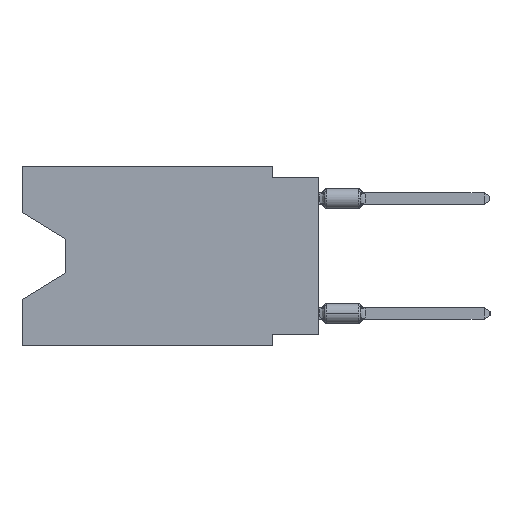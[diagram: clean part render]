
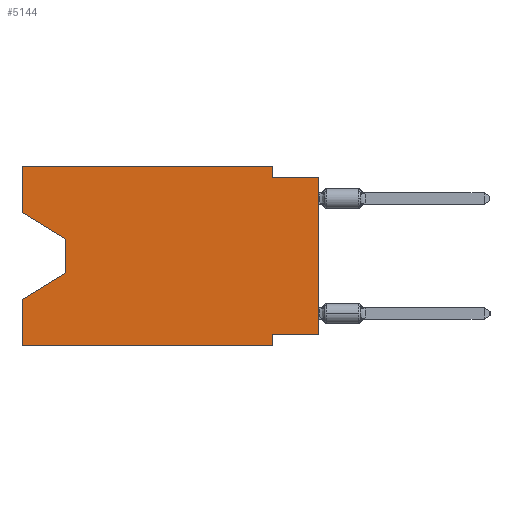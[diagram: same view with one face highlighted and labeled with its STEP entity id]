
A CAD part, left-side view. The second image highlights one B-rep face of the part: STEP entity #5144.
In plain terms, the highlighted planar face has unit normal (-1, 0, 0).
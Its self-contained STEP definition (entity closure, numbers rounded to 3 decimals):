
#274 = LINE ( 'NONE', #11532, #1977 ) ;
#690 = DIRECTION ( 'NONE',  ( 0., 0., -1. ) ) ;
#1440 = CARTESIAN_POINT ( 'NONE',  ( 0., 16.383, 0. ) ) ;
#1747 = VECTOR ( 'NONE', #36824, 1000. ) ;
#1977 = VECTOR ( 'NONE', #26783, 1000. ) ;
#3202 = EDGE_CURVE ( 'NONE', #27987, #41199, #40570, .T. ) ;
#3304 = LINE ( 'NONE', #14578, #1747 ) ;
#3527 = EDGE_CURVE ( 'NONE', #44847, #47909, #17283, .T. ) ;
#3804 = CARTESIAN_POINT ( 'NONE',  ( 0., 16.383, -7.36 ) ) ;
#4261 = VERTEX_POINT ( 'NONE', #49409 ) ;
#4263 = DIRECTION ( 'NONE',  ( 1., 0., 0. ) ) ;
#5144 = ADVANCED_FACE ( 'NONE', ( #42731 ), #8276, .F. ) ;
#5632 = EDGE_CURVE ( 'NONE', #35108, #4261, #16679, .T. ) ;
#5953 = CARTESIAN_POINT ( 'NONE',  ( 0., 16.383, -2.546 ) ) ;
#6007 = ORIENTED_EDGE ( 'NONE', *, *, #3527, .T. ) ;
#6340 = DIRECTION ( 'NONE',  ( 0., 0.855, -0.519 ) ) ;
#6975 = VERTEX_POINT ( 'NONE', #19221 ) ;
#7134 = ORIENTED_EDGE ( 'NONE', *, *, #3202, .T. ) ;
#7658 = EDGE_CURVE ( 'NONE', #43015, #47909, #18131, .T. ) ;
#8276 = PLANE ( 'NONE',  #19387 ) ;
#8695 = ORIENTED_EDGE ( 'NONE', *, *, #27275, .F. ) ;
#9591 = DIRECTION ( 'NONE',  ( 0., 0., 1. ) ) ;
#10071 = DIRECTION ( 'NONE',  ( 0., -1., 0. ) ) ;
#10151 = CARTESIAN_POINT ( 'NONE',  ( 0., 0., -0.635 ) ) ;
#10322 = CARTESIAN_POINT ( 'NONE',  ( 0., 2.54, 0. ) ) ;
#10509 = VECTOR ( 'NONE', #36534, 1000. ) ;
#11367 = CARTESIAN_POINT ( 'NONE',  ( 0., 2.54, -0.635 ) ) ;
#11532 = CARTESIAN_POINT ( 'NONE',  ( 0., 0., -9.271 ) ) ;
#12652 = VECTOR ( 'NONE', #44553, 1000. ) ;
#13189 = DIRECTION ( 'NONE',  ( 0., -1., 0. ) ) ;
#13385 = VECTOR ( 'NONE', #35360, 1000. ) ;
#13936 = CARTESIAN_POINT ( 'NONE',  ( 0., 16.383, -9.906 ) ) ;
#14056 = VERTEX_POINT ( 'NONE', #26756 ) ;
#14578 = CARTESIAN_POINT ( 'NONE',  ( 0., 16.383, 0. ) ) ;
#15410 = VECTOR ( 'NONE', #47177, 1000. ) ;
#15862 = ORIENTED_EDGE ( 'NONE', *, *, #24168, .T. ) ;
#16679 = LINE ( 'NONE', #47900, #18632 ) ;
#17283 = LINE ( 'NONE', #47758, #10509 ) ;
#17324 = CARTESIAN_POINT ( 'NONE',  ( 0., 2.54, 0. ) ) ;
#17822 = LINE ( 'NONE', #44307, #26389 ) ;
#17897 = DIRECTION ( 'NONE',  ( 0., -1., 0. ) ) ;
#18131 = LINE ( 'NONE', #10151, #45572 ) ;
#18632 = VECTOR ( 'NONE', #13189, 1000. ) ;
#19221 = CARTESIAN_POINT ( 'NONE',  ( 0., 16.383, -2.546 ) ) ;
#19224 = EDGE_CURVE ( 'NONE', #35108, #41199, #3304, .T. ) ;
#19387 = AXIS2_PLACEMENT_3D ( 'NONE', #23268, #4263, #34747 ) ;
#19467 = LINE ( 'NONE', #45941, #46322 ) ;
#20678 = EDGE_LOOP ( 'NONE', ( #21800, #15862, #7134, #25064, #30309, #8695, #37557, #6007, #38509, #37271, #46786, #31112 ) ) ;
#20855 = CARTESIAN_POINT ( 'NONE',  ( 0., 13.97, -5.893 ) ) ;
#20895 = EDGE_CURVE ( 'NONE', #6975, #33526, #36107, .T. ) ;
#21800 = ORIENTED_EDGE ( 'NONE', *, *, #30706, .T. ) ;
#21839 = LINE ( 'NONE', #22571, #12652 ) ;
#21880 = CARTESIAN_POINT ( 'NONE',  ( 0., 13.97, -5.893 ) ) ;
#22571 = CARTESIAN_POINT ( 'NONE',  ( 0., 13.97, -4.013 ) ) ;
#23268 = CARTESIAN_POINT ( 'NONE',  ( 0., 16.383, 0. ) ) ;
#24168 = EDGE_CURVE ( 'NONE', #44461, #27987, #21839, .T. ) ;
#25064 = ORIENTED_EDGE ( 'NONE', *, *, #19224, .F. ) ;
#26389 = VECTOR ( 'NONE', #10071, 1000. ) ;
#26553 = EDGE_CURVE ( 'NONE', #33526, #48408, #17822, .T. ) ;
#26756 = CARTESIAN_POINT ( 'NONE',  ( 0., 2.54, -9.271 ) ) ;
#26783 = DIRECTION ( 'NONE',  ( 0., 1., 0. ) ) ;
#27275 = EDGE_CURVE ( 'NONE', #14056, #4261, #19467, .T. ) ;
#27987 = VERTEX_POINT ( 'NONE', #21880 ) ;
#28346 = LINE ( 'NONE', #17324, #13385 ) ;
#30309 = ORIENTED_EDGE ( 'NONE', *, *, #5632, .T. ) ;
#30706 = EDGE_CURVE ( 'NONE', #6975, #44461, #43435, .T. ) ;
#31112 = ORIENTED_EDGE ( 'NONE', *, *, #20895, .F. ) ;
#32634 = CARTESIAN_POINT ( 'NONE',  ( 0., 0., -0.635 ) ) ;
#33042 = EDGE_CURVE ( 'NONE', #44847, #14056, #274, .T. ) ;
#33526 = VERTEX_POINT ( 'NONE', #1440 ) ;
#34747 = DIRECTION ( 'NONE',  ( 0., 0., -1. ) ) ;
#35108 = VERTEX_POINT ( 'NONE', #13936 ) ;
#35360 = DIRECTION ( 'NONE',  ( 0., 0., -1. ) ) ;
#36107 = LINE ( 'NONE', #43822, #39268 ) ;
#36534 = DIRECTION ( 'NONE',  ( 0., 0., 1. ) ) ;
#36824 = DIRECTION ( 'NONE',  ( 0., 0., 1. ) ) ;
#37271 = ORIENTED_EDGE ( 'NONE', *, *, #43102, .F. ) ;
#37557 = ORIENTED_EDGE ( 'NONE', *, *, #33042, .F. ) ;
#38509 = ORIENTED_EDGE ( 'NONE', *, *, #7658, .F. ) ;
#39268 = VECTOR ( 'NONE', #9591, 1000. ) ;
#40570 = LINE ( 'NONE', #20855, #46340 ) ;
#41199 = VERTEX_POINT ( 'NONE', #3804 ) ;
#42731 = FACE_OUTER_BOUND ( 'NONE', #20678, .T. ) ;
#43015 = VERTEX_POINT ( 'NONE', #11367 ) ;
#43102 = EDGE_CURVE ( 'NONE', #48408, #43015, #28346, .T. ) ;
#43435 = LINE ( 'NONE', #5953, #15410 ) ;
#43767 = CARTESIAN_POINT ( 'NONE',  ( 0., 0., -9.271 ) ) ;
#43822 = CARTESIAN_POINT ( 'NONE',  ( 0., 16.383, 0. ) ) ;
#44307 = CARTESIAN_POINT ( 'NONE',  ( 0., 16.383, 0. ) ) ;
#44461 = VERTEX_POINT ( 'NONE', #44558 ) ;
#44553 = DIRECTION ( 'NONE',  ( 0., 0., -1. ) ) ;
#44558 = CARTESIAN_POINT ( 'NONE',  ( 0., 13.97, -4.013 ) ) ;
#44847 = VERTEX_POINT ( 'NONE', #43767 ) ;
#45572 = VECTOR ( 'NONE', #17897, 1000. ) ;
#45941 = CARTESIAN_POINT ( 'NONE',  ( 0., 2.54, -9.906 ) ) ;
#46322 = VECTOR ( 'NONE', #690, 1000. ) ;
#46340 = VECTOR ( 'NONE', #6340, 1000. ) ;
#46786 = ORIENTED_EDGE ( 'NONE', *, *, #26553, .F. ) ;
#47177 = DIRECTION ( 'NONE',  ( 0., -0.855, -0.519 ) ) ;
#47758 = CARTESIAN_POINT ( 'NONE',  ( 0., 0., 0. ) ) ;
#47900 = CARTESIAN_POINT ( 'NONE',  ( 0., 16.383, -9.906 ) ) ;
#47909 = VERTEX_POINT ( 'NONE', #32634 ) ;
#48408 = VERTEX_POINT ( 'NONE', #10322 ) ;
#49409 = CARTESIAN_POINT ( 'NONE',  ( 0., 2.54, -9.906 ) ) ;
